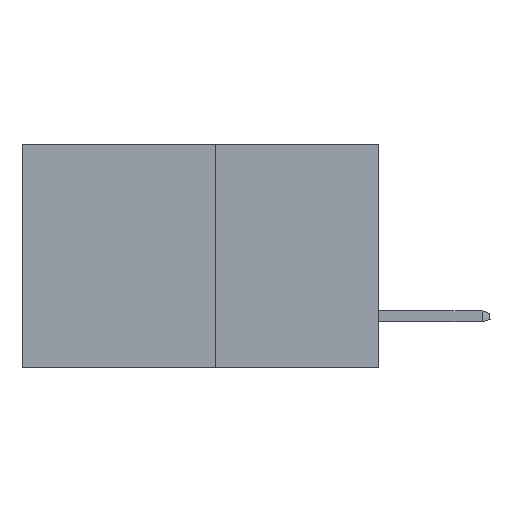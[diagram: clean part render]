
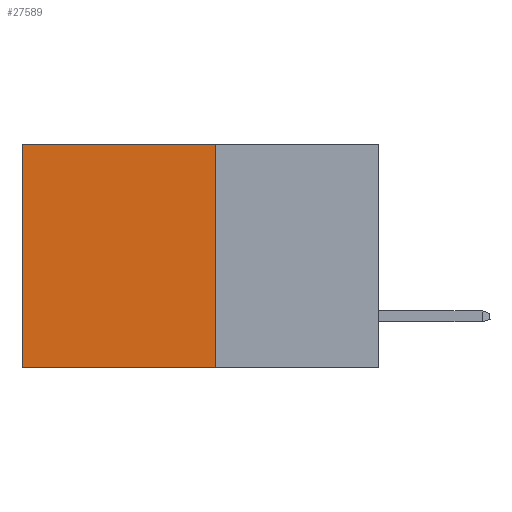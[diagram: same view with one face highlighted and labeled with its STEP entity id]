
A CAD part, left-side view. The second image highlights one B-rep face of the part: STEP entity #27589.
In plain terms, the highlighted planar face has unit normal (-1, 0, 0).
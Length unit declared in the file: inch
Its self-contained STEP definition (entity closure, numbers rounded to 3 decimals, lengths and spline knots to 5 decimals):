
#255 = EDGE_LOOP ( 'NONE', ( #1572, #22679, #1018, #15158 ) ) ;
#1018 = ORIENTED_EDGE ( 'NONE', *, *, #5746, .F. ) ;
#1461 = LINE ( 'NONE', #12642, #19961 ) ;
#1572 = ORIENTED_EDGE ( 'NONE', *, *, #25618, .T. ) ;
#1794 = DIRECTION ( 'NONE',  ( 0., 1., 0. ) ) ;
#2186 = CARTESIAN_POINT ( 'NONE',  ( 0.277, 0.59, 0. ) ) ;
#3433 = VECTOR ( 'NONE', #3775, 39.37008 ) ;
#3775 = DIRECTION ( 'NONE',  ( 0., 0., -1. ) ) ;
#5180 = VERTEX_POINT ( 'NONE', #12463 ) ;
#5746 = EDGE_CURVE ( 'NONE', #13143, #5180, #1461, .T. ) ;
#5944 = VECTOR ( 'NONE', #27971, 39.37008 ) ;
#10098 = DIRECTION ( 'NONE',  ( 0., 0., -1. ) ) ;
#11602 = PLANE ( 'NONE',  #27421 ) ;
#12463 = CARTESIAN_POINT ( 'NONE',  ( 0.277, 0.27, -0.37 ) ) ;
#12642 = CARTESIAN_POINT ( 'NONE',  ( 0.277, 0.27, -0.37 ) ) ;
#12669 = LINE ( 'NONE', #13012, #5944 ) ;
#13012 = CARTESIAN_POINT ( 'NONE',  ( 0.277, 0.27, -0.37 ) ) ;
#13143 = VERTEX_POINT ( 'NONE', #28294 ) ;
#14133 = DIRECTION ( 'NONE',  ( 0., 0., -1. ) ) ;
#15158 = ORIENTED_EDGE ( 'NONE', *, *, #21104, .T. ) ;
#16331 = CARTESIAN_POINT ( 'NONE',  ( 0.277, 0.59, -0.37 ) ) ;
#16580 = VERTEX_POINT ( 'NONE', #2186 ) ;
#16767 = FACE_OUTER_BOUND ( 'NONE', #255, .T. ) ;
#16798 = CARTESIAN_POINT ( 'NONE',  ( 0.277, 0.27, 0. ) ) ;
#19609 = CARTESIAN_POINT ( 'NONE',  ( 0.277, 0.59, -0.37 ) ) ;
#19961 = VECTOR ( 'NONE', #10098, 39.37008 ) ;
#20798 = LINE ( 'NONE', #16798, #26621 ) ;
#21104 = EDGE_CURVE ( 'NONE', #13143, #16580, #20798, .T. ) ;
#22679 = ORIENTED_EDGE ( 'NONE', *, *, #23989, .F. ) ;
#23421 = LINE ( 'NONE', #16331, #3433 ) ;
#23989 = EDGE_CURVE ( 'NONE', #5180, #27727, #12669, .T. ) ;
#24051 = CARTESIAN_POINT ( 'NONE',  ( 0.277, 0.27, -0.37 ) ) ;
#25618 = EDGE_CURVE ( 'NONE', #16580, #27727, #23421, .T. ) ;
#26621 = VECTOR ( 'NONE', #1794, 39.37008 ) ;
#27421 = AXIS2_PLACEMENT_3D ( 'NONE', #24051, #29102, #14133 ) ;
#27589 = ADVANCED_FACE ( 'NONE', ( #16767 ), #11602, .F. ) ;
#27727 = VERTEX_POINT ( 'NONE', #19609 ) ;
#27971 = DIRECTION ( 'NONE',  ( 0., 1., 0. ) ) ;
#28294 = CARTESIAN_POINT ( 'NONE',  ( 0.277, 0.27, 0. ) ) ;
#29102 = DIRECTION ( 'NONE',  ( 1., 0., 0. ) ) ;
